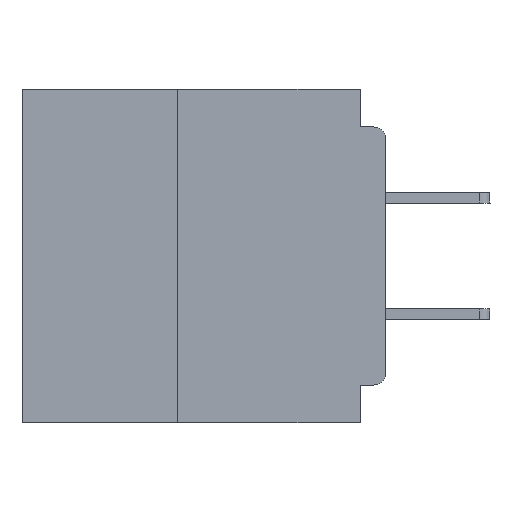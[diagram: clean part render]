
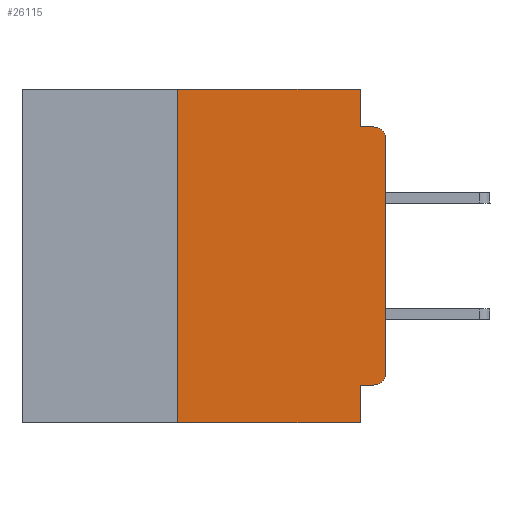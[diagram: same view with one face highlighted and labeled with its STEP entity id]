
A CAD part, left-side view. The second image highlights one B-rep face of the part: STEP entity #26115.
In plain terms, the highlighted planar face has unit normal (-1, 0, 0).
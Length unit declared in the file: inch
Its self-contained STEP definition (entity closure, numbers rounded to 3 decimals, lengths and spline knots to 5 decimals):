
#179 = ORIENTED_EDGE ( 'NONE', *, *, #18480, .T. ) ;
#2237 = EDGE_LOOP ( 'NONE', ( #37425, #32971, #10564, #3082, #47190, #24579, #179, #10886, #9430, #24793 ) ) ;
#3082 = ORIENTED_EDGE ( 'NONE', *, *, #45845, .F. ) ;
#4218 = EDGE_CURVE ( 'NONE', #10976, #61249, #13339, .T. ) ;
#4242 = DIRECTION ( 'NONE',  ( -1., 0., 0. ) ) ;
#7700 = CARTESIAN_POINT ( 'NONE',  ( 0., 0.031, -0.4 ) ) ;
#9430 = ORIENTED_EDGE ( 'NONE', *, *, #60898, .F. ) ;
#10564 = ORIENTED_EDGE ( 'NONE', *, *, #67768, .F. ) ;
#10886 = ORIENTED_EDGE ( 'NONE', *, *, #24862, .F. ) ;
#10976 = VERTEX_POINT ( 'NONE', #12995 ) ;
#11458 = DIRECTION ( 'NONE',  ( 0., -1., 0. ) ) ;
#12864 = VERTEX_POINT ( 'NONE', #7700 ) ;
#12995 = CARTESIAN_POINT ( 'NONE',  ( 0., 0.25, -0.4 ) ) ;
#13339 = LINE ( 'NONE', #54624, #67834 ) ;
#13690 = CARTESIAN_POINT ( 'NONE',  ( 0., 0.437, 0. ) ) ;
#13970 = CARTESIAN_POINT ( 'NONE',  ( 0., 0.031, 0. ) ) ;
#14772 = DIRECTION ( 'NONE',  ( 0., 0., 1. ) ) ;
#16639 = VECTOR ( 'NONE', #11458, 39.37008 ) ;
#17316 = CARTESIAN_POINT ( 'NONE',  ( 0., 0.031, 0. ) ) ;
#18480 = EDGE_CURVE ( 'NONE', #10976, #12864, #30720, .T. ) ;
#19249 = CARTESIAN_POINT ( 'NONE',  ( 0., 0.015, -0.06 ) ) ;
#19704 = VECTOR ( 'NONE', #31096, 39.37008 ) ;
#19891 = CARTESIAN_POINT ( 'NONE',  ( 0., 0., 0. ) ) ;
#20204 = CARTESIAN_POINT ( 'NONE',  ( 0., 0., -0.045 ) ) ;
#20893 = CARTESIAN_POINT ( 'NONE',  ( 0., 0., -0.06 ) ) ;
#21065 = DIRECTION ( 'NONE',  ( 0., 1., 0. ) ) ;
#21384 = LINE ( 'NONE', #47048, #19704 ) ;
#21578 = VERTEX_POINT ( 'NONE', #41818 ) ;
#22278 = AXIS2_PLACEMENT_3D ( 'NONE', #36012, #4242, #41341 ) ;
#22473 = VERTEX_POINT ( 'NONE', #54343 ) ;
#24336 = DIRECTION ( 'NONE',  ( 1., 0., 0. ) ) ;
#24540 = DIRECTION ( 'NONE',  ( 0., 0., -1. ) ) ;
#24579 = ORIENTED_EDGE ( 'NONE', *, *, #4218, .F. ) ;
#24793 = ORIENTED_EDGE ( 'NONE', *, *, #28698, .T. ) ;
#24862 = EDGE_CURVE ( 'NONE', #22473, #12864, #29358, .T. ) ;
#25873 = AXIS2_PLACEMENT_3D ( 'NONE', #19249, #56187, #24540 ) ;
#26115 = ADVANCED_FACE ( 'NONE', ( #33432 ), #50657, .F. ) ;
#26328 = VECTOR ( 'NONE', #21065, 39.37008 ) ;
#28138 = CARTESIAN_POINT ( 'NONE',  ( 0., 0.25, 0. ) ) ;
#28698 = EDGE_CURVE ( 'NONE', #49303, #35304, #31371, .T. ) ;
#29358 = LINE ( 'NONE', #34932, #55788 ) ;
#29507 = LINE ( 'NONE', #20204, #41966 ) ;
#30720 = LINE ( 'NONE', #53312, #16639 ) ;
#31096 = DIRECTION ( 'NONE',  ( 0., -1., 0. ) ) ;
#31371 = CIRCLE ( 'NONE', #22278, 0.015 ) ;
#32971 = ORIENTED_EDGE ( 'NONE', *, *, #58654, .T. ) ;
#33432 = FACE_OUTER_BOUND ( 'NONE', #2237, .T. ) ;
#34680 = CIRCLE ( 'NONE', #25873, 0.015 ) ;
#34932 = CARTESIAN_POINT ( 'NONE',  ( 0., 0.031, -0.4 ) ) ;
#35304 = VERTEX_POINT ( 'NONE', #61044 ) ;
#35930 = EDGE_CURVE ( 'NONE', #35304, #49952, #59501, .T. ) ;
#36012 = CARTESIAN_POINT ( 'NONE',  ( 0., 0.015, -0.34 ) ) ;
#37425 = ORIENTED_EDGE ( 'NONE', *, *, #35930, .T. ) ;
#39007 = DIRECTION ( 'NONE',  ( 0., 0., 1. ) ) ;
#39565 = CARTESIAN_POINT ( 'NONE',  ( 0., 0.015, -0.045 ) ) ;
#41341 = DIRECTION ( 'NONE',  ( 0., 0., -1. ) ) ;
#41818 = CARTESIAN_POINT ( 'NONE',  ( 0., 0.031, -0.045 ) ) ;
#41966 = VECTOR ( 'NONE', #51838, 39.37008 ) ;
#45492 = VECTOR ( 'NONE', #14772, 39.37008 ) ;
#45845 = EDGE_CURVE ( 'NONE', #66323, #21578, #64037, .T. ) ;
#47048 = CARTESIAN_POINT ( 'NONE',  ( 0., 0.437, 0. ) ) ;
#47190 = ORIENTED_EDGE ( 'NONE', *, *, #49130, .F. ) ;
#49130 = EDGE_CURVE ( 'NONE', #61249, #66323, #21384, .T. ) ;
#49303 = VERTEX_POINT ( 'NONE', #64280 ) ;
#49952 = VERTEX_POINT ( 'NONE', #20893 ) ;
#50657 = PLANE ( 'NONE',  #61091 ) ;
#51838 = DIRECTION ( 'NONE',  ( 0., -1., 0. ) ) ;
#53312 = CARTESIAN_POINT ( 'NONE',  ( 0., 0.437, -0.4 ) ) ;
#54343 = CARTESIAN_POINT ( 'NONE',  ( 0., 0.031, -0.355 ) ) ;
#54624 = CARTESIAN_POINT ( 'NONE',  ( 0., 0.25, -0.4 ) ) ;
#55788 = VECTOR ( 'NONE', #56141, 39.37008 ) ;
#56141 = DIRECTION ( 'NONE',  ( 0., 0., -1. ) ) ;
#56187 = DIRECTION ( 'NONE',  ( -1., 0., 0. ) ) ;
#56481 = DIRECTION ( 'NONE',  ( 0., 0., -1. ) ) ;
#58113 = VERTEX_POINT ( 'NONE', #39565 ) ;
#58654 = EDGE_CURVE ( 'NONE', #49952, #58113, #34680, .T. ) ;
#59501 = LINE ( 'NONE', #19891, #45492 ) ;
#60898 = EDGE_CURVE ( 'NONE', #49303, #22473, #68411, .T. ) ;
#61044 = CARTESIAN_POINT ( 'NONE',  ( 0., 0., -0.34 ) ) ;
#61091 = AXIS2_PLACEMENT_3D ( 'NONE', #13690, #24336, #61288 ) ;
#61249 = VERTEX_POINT ( 'NONE', #28138 ) ;
#61288 = DIRECTION ( 'NONE',  ( 0., 0., -1. ) ) ;
#62393 = VECTOR ( 'NONE', #56481, 39.37008 ) ;
#64037 = LINE ( 'NONE', #13970, #62393 ) ;
#64280 = CARTESIAN_POINT ( 'NONE',  ( 0., 0.015, -0.355 ) ) ;
#66323 = VERTEX_POINT ( 'NONE', #17316 ) ;
#67768 = EDGE_CURVE ( 'NONE', #21578, #58113, #29507, .T. ) ;
#67834 = VECTOR ( 'NONE', #39007, 39.37008 ) ;
#68319 = CARTESIAN_POINT ( 'NONE',  ( 0., 0., -0.355 ) ) ;
#68411 = LINE ( 'NONE', #68319, #26328 ) ;
